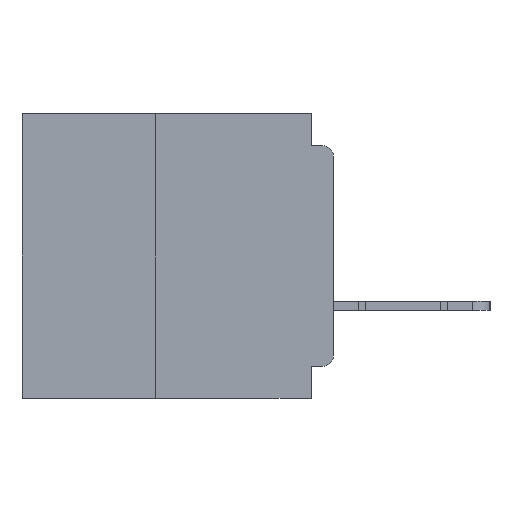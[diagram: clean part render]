
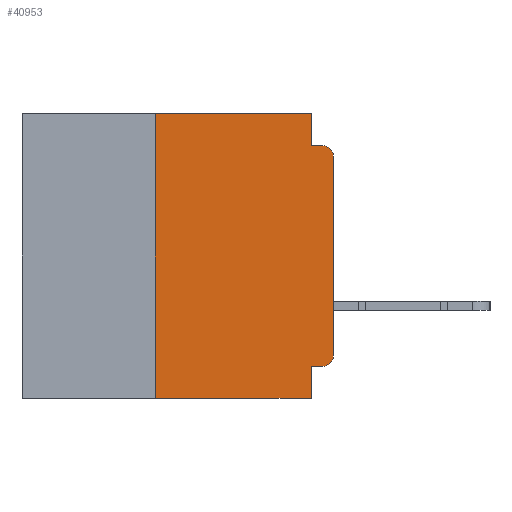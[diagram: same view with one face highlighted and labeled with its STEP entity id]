
A CAD part, left-side view. The second image highlights one B-rep face of the part: STEP entity #40953.
In plain terms, the highlighted planar face has unit normal (-1, 0, 0).
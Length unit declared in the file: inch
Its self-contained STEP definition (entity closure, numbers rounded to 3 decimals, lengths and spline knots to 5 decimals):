
#62 = DIRECTION ( 'NONE',  ( 0., 0., -1. ) ) ;
#66 = CARTESIAN_POINT ( 'NONE',  ( 0., 0.031, 0. ) ) ;
#288 = FACE_OUTER_BOUND ( 'NONE', #48862, .T. ) ;
#865 = CARTESIAN_POINT ( 'NONE',  ( 0., 0.031, -0.045 ) ) ;
#1254 = ORIENTED_EDGE ( 'NONE', *, *, #43061, .T. ) ;
#2692 = VECTOR ( 'NONE', #54135, 39.37008 ) ;
#3024 = CARTESIAN_POINT ( 'NONE',  ( 0., 0.015, -0.045 ) ) ;
#3085 = VERTEX_POINT ( 'NONE', #30958 ) ;
#3773 = DIRECTION ( 'NONE',  ( 0., 0., -1. ) ) ;
#4388 = LINE ( 'NONE', #5857, #2692 ) ;
#4395 = EDGE_CURVE ( 'NONE', #56765, #16635, #4388, .T. ) ;
#5555 = CARTESIAN_POINT ( 'NONE',  ( 0., 0.031, -0.4 ) ) ;
#5857 = CARTESIAN_POINT ( 'NONE',  ( 0., 0.031, 0. ) ) ;
#6683 = EDGE_CURVE ( 'NONE', #27799, #32491, #47690, .T. ) ;
#8752 = CARTESIAN_POINT ( 'NONE',  ( 0., 0.015, -0.34 ) ) ;
#10422 = ORIENTED_EDGE ( 'NONE', *, *, #10655, .F. ) ;
#10655 = EDGE_CURVE ( 'NONE', #62743, #56765, #47056, .T. ) ;
#11112 = CIRCLE ( 'NONE', #51564, 0.015 ) ;
#11858 = CARTESIAN_POINT ( 'NONE',  ( 0., 0., -0.06 ) ) ;
#12566 = CARTESIAN_POINT ( 'NONE',  ( 0., 0., 0. ) ) ;
#13088 = VECTOR ( 'NONE', #65862, 39.37008 ) ;
#13955 = VECTOR ( 'NONE', #55769, 39.37008 ) ;
#14213 = DIRECTION ( 'NONE',  ( 0., 0., -1. ) ) ;
#14706 = EDGE_CURVE ( 'NONE', #16635, #53446, #17079, .T. ) ;
#15440 = EDGE_CURVE ( 'NONE', #3085, #62743, #66283, .T. ) ;
#16635 = VERTEX_POINT ( 'NONE', #865 ) ;
#16681 = DIRECTION ( 'NONE',  ( 0., 0., 1. ) ) ;
#17079 = LINE ( 'NONE', #26131, #43874 ) ;
#17483 = DIRECTION ( 'NONE',  ( 0., -1., 0. ) ) ;
#18345 = CARTESIAN_POINT ( 'NONE',  ( 0., 0., -0.355 ) ) ;
#20161 = DIRECTION ( 'NONE',  ( 1., 0., 0. ) ) ;
#20835 = ORIENTED_EDGE ( 'NONE', *, *, #47254, .T. ) ;
#21868 = CARTESIAN_POINT ( 'NONE',  ( 0., 0.015, -0.355 ) ) ;
#21891 = VECTOR ( 'NONE', #31200, 39.37008 ) ;
#26131 = CARTESIAN_POINT ( 'NONE',  ( 0., 0., -0.045 ) ) ;
#27799 = VERTEX_POINT ( 'NONE', #46077 ) ;
#30479 = ORIENTED_EDGE ( 'NONE', *, *, #68652, .T. ) ;
#30492 = AXIS2_PLACEMENT_3D ( 'NONE', #30709, #20161, #57598 ) ;
#30709 = CARTESIAN_POINT ( 'NONE',  ( 0., 0.437, 0. ) ) ;
#30958 = CARTESIAN_POINT ( 'NONE',  ( 0., 0.25, -0.4 ) ) ;
#31199 = VERTEX_POINT ( 'NONE', #21868 ) ;
#31200 = DIRECTION ( 'NONE',  ( 0., -1., 0. ) ) ;
#32491 = VERTEX_POINT ( 'NONE', #49577 ) ;
#33459 = VECTOR ( 'NONE', #62, 39.37008 ) ;
#33527 = VERTEX_POINT ( 'NONE', #11858 ) ;
#35998 = DIRECTION ( 'NONE',  ( -1., 0., 0. ) ) ;
#38763 = CARTESIAN_POINT ( 'NONE',  ( 0., 0.25, 0. ) ) ;
#38789 = CARTESIAN_POINT ( 'NONE',  ( 0., 0.437, -0.4 ) ) ;
#39547 = VECTOR ( 'NONE', #17483, 39.37008 ) ;
#40775 = LINE ( 'NONE', #18345, #13955 ) ;
#40953 = ADVANCED_FACE ( 'NONE', ( #288 ), #52202, .F. ) ;
#41238 = LINE ( 'NONE', #38789, #39547 ) ;
#41621 = LINE ( 'NONE', #12566, #13088 ) ;
#43061 = EDGE_CURVE ( 'NONE', #3085, #32491, #41238, .T. ) ;
#43874 = VECTOR ( 'NONE', #47679, 39.37008 ) ;
#44275 = AXIS2_PLACEMENT_3D ( 'NONE', #67891, #35998, #3773 ) ;
#46077 = CARTESIAN_POINT ( 'NONE',  ( 0., 0.031, -0.355 ) ) ;
#46292 = DIRECTION ( 'NONE',  ( -1., 0., 0. ) ) ;
#47056 = LINE ( 'NONE', #63195, #21891 ) ;
#47254 = EDGE_CURVE ( 'NONE', #54552, #33527, #41621, .T. ) ;
#47679 = DIRECTION ( 'NONE',  ( 0., -1., 0. ) ) ;
#47690 = LINE ( 'NONE', #5555, #33459 ) ;
#48374 = ORIENTED_EDGE ( 'NONE', *, *, #6683, .F. ) ;
#48750 = CARTESIAN_POINT ( 'NONE',  ( 0., 0.25, -0.4 ) ) ;
#48862 = EDGE_LOOP ( 'NONE', ( #20835, #67659, #55003, #66729, #10422, #54538, #1254, #48374, #64387, #30479 ) ) ;
#49577 = CARTESIAN_POINT ( 'NONE',  ( 0., 0.031, -0.4 ) ) ;
#50409 = EDGE_CURVE ( 'NONE', #31199, #27799, #40775, .T. ) ;
#51564 = AXIS2_PLACEMENT_3D ( 'NONE', #8752, #46292, #14213 ) ;
#52139 = VECTOR ( 'NONE', #16681, 39.37008 ) ;
#52202 = PLANE ( 'NONE',  #30492 ) ;
#53446 = VERTEX_POINT ( 'NONE', #3024 ) ;
#54135 = DIRECTION ( 'NONE',  ( 0., 0., -1. ) ) ;
#54538 = ORIENTED_EDGE ( 'NONE', *, *, #15440, .F. ) ;
#54552 = VERTEX_POINT ( 'NONE', #60061 ) ;
#55003 = ORIENTED_EDGE ( 'NONE', *, *, #14706, .F. ) ;
#55769 = DIRECTION ( 'NONE',  ( 0., 1., 0. ) ) ;
#56765 = VERTEX_POINT ( 'NONE', #66 ) ;
#57598 = DIRECTION ( 'NONE',  ( 0., 0., -1. ) ) ;
#60061 = CARTESIAN_POINT ( 'NONE',  ( 0., 0., -0.34 ) ) ;
#62743 = VERTEX_POINT ( 'NONE', #38763 ) ;
#63195 = CARTESIAN_POINT ( 'NONE',  ( 0., 0.437, 0. ) ) ;
#64387 = ORIENTED_EDGE ( 'NONE', *, *, #50409, .F. ) ;
#65862 = DIRECTION ( 'NONE',  ( 0., 0., 1. ) ) ;
#66283 = LINE ( 'NONE', #48750, #52139 ) ;
#66361 = EDGE_CURVE ( 'NONE', #33527, #53446, #67023, .T. ) ;
#66729 = ORIENTED_EDGE ( 'NONE', *, *, #4395, .F. ) ;
#67023 = CIRCLE ( 'NONE', #44275, 0.015 ) ;
#67659 = ORIENTED_EDGE ( 'NONE', *, *, #66361, .T. ) ;
#67891 = CARTESIAN_POINT ( 'NONE',  ( 0., 0.015, -0.06 ) ) ;
#68652 = EDGE_CURVE ( 'NONE', #31199, #54552, #11112, .T. ) ;
